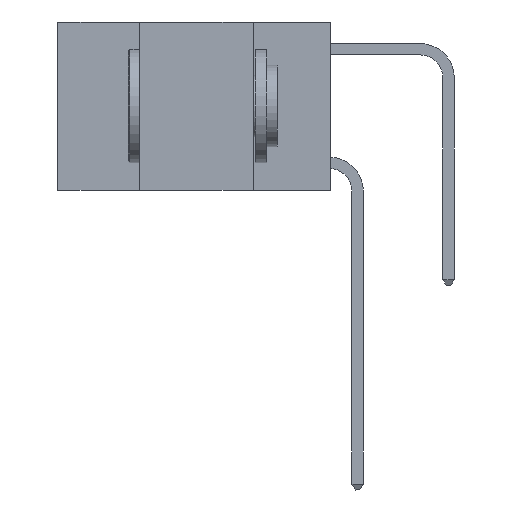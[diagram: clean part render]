
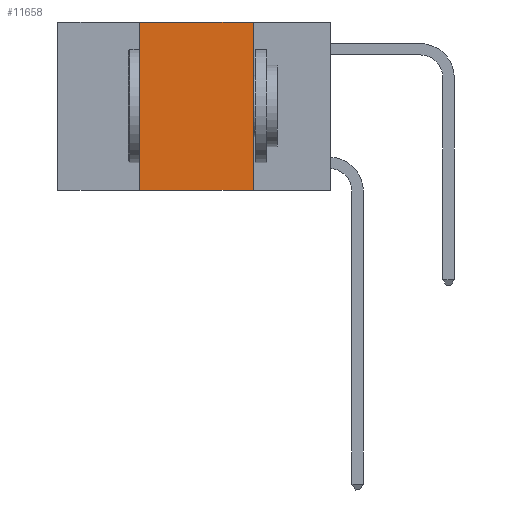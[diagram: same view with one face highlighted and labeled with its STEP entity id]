
A CAD part, left-side view. The second image highlights one B-rep face of the part: STEP entity #11658.
In plain terms, the highlighted planar face has unit normal (-1, 0, 0).
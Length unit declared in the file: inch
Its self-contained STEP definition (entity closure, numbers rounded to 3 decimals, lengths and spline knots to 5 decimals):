
#92 = DIRECTION ( 'NONE',  ( 0., 0., -1. ) ) ;
#400 = CARTESIAN_POINT ( 'NONE',  ( 0., 0.17, -0.37 ) ) ;
#544 = CARTESIAN_POINT ( 'NONE',  ( 0., 0.42, 0. ) ) ;
#1042 = LINE ( 'NONE', #9316, #10430 ) ;
#1340 = AXIS2_PLACEMENT_3D ( 'NONE', #5809, #9428, #92 ) ;
#1662 = LINE ( 'NONE', #1730, #11412 ) ;
#1730 = CARTESIAN_POINT ( 'NONE',  ( 0., 0.6, 0. ) ) ;
#2579 = LINE ( 'NONE', #544, #11223 ) ;
#2751 = CARTESIAN_POINT ( 'NONE',  ( 0., 0.17, 0. ) ) ;
#3310 = EDGE_CURVE ( 'NONE', #5041, #10824, #1042, .T. ) ;
#3675 = DIRECTION ( 'NONE',  ( 0., -1., 0. ) ) ;
#3840 = ORIENTED_EDGE ( 'NONE', *, *, #3310, .F. ) ;
#3856 = EDGE_LOOP ( 'NONE', ( #3840, #6486, #6172, #7631 ) ) ;
#5041 = VERTEX_POINT ( 'NONE', #2751 ) ;
#5153 = CARTESIAN_POINT ( 'NONE',  ( 0., 0.42, 0. ) ) ;
#5300 = EDGE_CURVE ( 'NONE', #9588, #5041, #1662, .T. ) ;
#5580 = EDGE_CURVE ( 'NONE', #6484, #10824, #10512, .T. ) ;
#5627 = CARTESIAN_POINT ( 'NONE',  ( 0., 0.6, -0.37 ) ) ;
#5809 = CARTESIAN_POINT ( 'NONE',  ( 0., 0.6, 0. ) ) ;
#6172 = ORIENTED_EDGE ( 'NONE', *, *, #7570, .F. ) ;
#6372 = DIRECTION ( 'NONE',  ( 0., 0., 1. ) ) ;
#6484 = VERTEX_POINT ( 'NONE', #10379 ) ;
#6486 = ORIENTED_EDGE ( 'NONE', *, *, #5300, .F. ) ;
#7570 = EDGE_CURVE ( 'NONE', #6484, #9588, #2579, .T. ) ;
#7631 = ORIENTED_EDGE ( 'NONE', *, *, #5580, .T. ) ;
#7718 = FACE_OUTER_BOUND ( 'NONE', #3856, .T. ) ;
#8625 = DIRECTION ( 'NONE',  ( 0., 0., -1. ) ) ;
#9316 = CARTESIAN_POINT ( 'NONE',  ( 0., 0.17, 0. ) ) ;
#9428 = DIRECTION ( 'NONE',  ( 1., 0., 0. ) ) ;
#9588 = VERTEX_POINT ( 'NONE', #5153 ) ;
#9676 = PLANE ( 'NONE',  #1340 ) ;
#10379 = CARTESIAN_POINT ( 'NONE',  ( 0., 0.42, -0.37 ) ) ;
#10430 = VECTOR ( 'NONE', #8625, 39.37008 ) ;
#10447 = DIRECTION ( 'NONE',  ( 0., -1., 0. ) ) ;
#10512 = LINE ( 'NONE', #5627, #11797 ) ;
#10824 = VERTEX_POINT ( 'NONE', #400 ) ;
#11223 = VECTOR ( 'NONE', #6372, 39.37008 ) ;
#11412 = VECTOR ( 'NONE', #3675, 39.37008 ) ;
#11658 = ADVANCED_FACE ( 'NONE', ( #7718 ), #9676, .F. ) ;
#11797 = VECTOR ( 'NONE', #10447, 39.37008 ) ;
